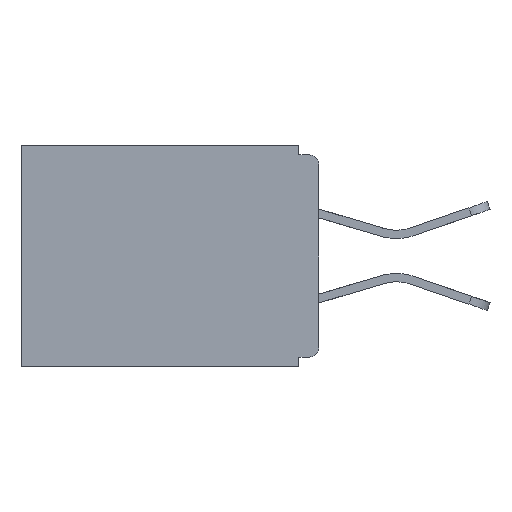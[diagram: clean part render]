
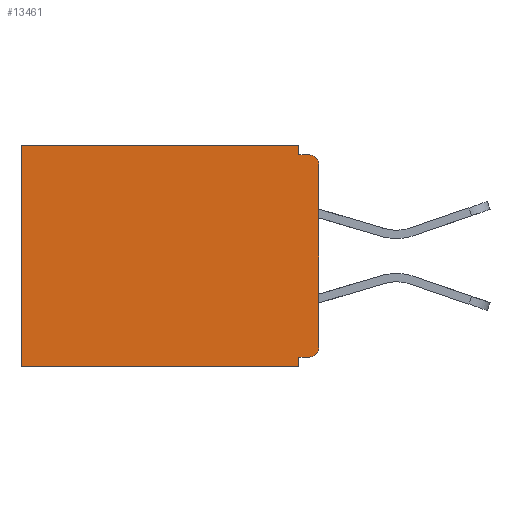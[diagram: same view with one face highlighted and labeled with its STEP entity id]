
A CAD part, left-side view. The second image highlights one B-rep face of the part: STEP entity #13461.
In plain terms, the highlighted planar face has unit normal (-1, 0, 0).
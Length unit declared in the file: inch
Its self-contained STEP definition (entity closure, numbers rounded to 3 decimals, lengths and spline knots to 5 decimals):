
#26 = CARTESIAN_POINT ( 'NONE',  ( 0.298, 0.031, -0.015 ) ) ;
#28 = CARTESIAN_POINT ( 'NONE',  ( 0.298, 0.031, -0.343 ) ) ;
#801 = ORIENTED_EDGE ( 'NONE', *, *, #3856, .F. ) ;
#1372 = CARTESIAN_POINT ( 'NONE',  ( 0.298, 0.015, -0.328 ) ) ;
#1725 = VERTEX_POINT ( 'NONE', #3124 ) ;
#2933 = LINE ( 'NONE', #20693, #17212 ) ;
#3124 = CARTESIAN_POINT ( 'NONE',  ( 0.298, 0., -0.313 ) ) ;
#3155 = DIRECTION ( 'NONE',  ( 1., 0., 0. ) ) ;
#3326 = DIRECTION ( 'NONE',  ( 0., 0., -1. ) ) ;
#3626 = ORIENTED_EDGE ( 'NONE', *, *, #18985, .F. ) ;
#3690 = LINE ( 'NONE', #6072, #11023 ) ;
#3773 = VERTEX_POINT ( 'NONE', #9510 ) ;
#3856 = EDGE_CURVE ( 'NONE', #18642, #16194, #2933, .T. ) ;
#3944 = CARTESIAN_POINT ( 'NONE',  ( 0.298, 0.46, 0. ) ) ;
#4284 = ORIENTED_EDGE ( 'NONE', *, *, #15803, .T. ) ;
#5026 = ORIENTED_EDGE ( 'NONE', *, *, #6242, .T. ) ;
#5992 = CARTESIAN_POINT ( 'NONE',  ( 0.298, 0.031, -0.328 ) ) ;
#6072 = CARTESIAN_POINT ( 'NONE',  ( 0.298, 0., -0.343 ) ) ;
#6242 = EDGE_CURVE ( 'NONE', #18642, #1725, #12892, .T. ) ;
#6780 = VECTOR ( 'NONE', #15890, 39.37008 ) ;
#7370 = LINE ( 'NONE', #23292, #15363 ) ;
#7506 = CARTESIAN_POINT ( 'NONE',  ( 0.298, 0.031, -0.343 ) ) ;
#8250 = AXIS2_PLACEMENT_3D ( 'NONE', #19083, #21010, #25500 ) ;
#8762 = ORIENTED_EDGE ( 'NONE', *, *, #12440, .T. ) ;
#9299 = CARTESIAN_POINT ( 'NONE',  ( 0.298, 0., 0. ) ) ;
#9510 = CARTESIAN_POINT ( 'NONE',  ( 0.298, 0.015, -0.015 ) ) ;
#9830 = EDGE_CURVE ( 'NONE', #27443, #1725, #27353, .T. ) ;
#9964 = VERTEX_POINT ( 'NONE', #25817 ) ;
#9993 = CARTESIAN_POINT ( 'NONE',  ( 0.298, 0.031, 0. ) ) ;
#10000 = CIRCLE ( 'NONE', #27553, 0.015 ) ;
#10158 = ORIENTED_EDGE ( 'NONE', *, *, #10792, .T. ) ;
#10476 = VECTOR ( 'NONE', #16691, 39.37008 ) ;
#10576 = AXIS2_PLACEMENT_3D ( 'NONE', #9299, #3155, #18013 ) ;
#10618 = DIRECTION ( 'NONE',  ( 0., 0., -1. ) ) ;
#10792 = EDGE_CURVE ( 'NONE', #27443, #3773, #10000, .T. ) ;
#10989 = VERTEX_POINT ( 'NONE', #3944 ) ;
#11023 = VECTOR ( 'NONE', #27179, 39.37008 ) ;
#11535 = PLANE ( 'NONE',  #10576 ) ;
#12085 = DIRECTION ( 'NONE',  ( -1., 0., 0. ) ) ;
#12440 = EDGE_CURVE ( 'NONE', #23164, #10989, #18532, .T. ) ;
#12633 = LINE ( 'NONE', #7506, #13975 ) ;
#12892 = CIRCLE ( 'NONE', #8250, 0.015 ) ;
#13461 = ADVANCED_FACE ( 'NONE', ( #26113 ), #11535, .F. ) ;
#13865 = CARTESIAN_POINT ( 'NONE',  ( 0.298, 0.015, -0.03 ) ) ;
#13975 = VECTOR ( 'NONE', #3326, 39.37008 ) ;
#14434 = LINE ( 'NONE', #26762, #6780 ) ;
#14671 = EDGE_CURVE ( 'NONE', #23164, #26048, #15767, .T. ) ;
#14679 = VERTEX_POINT ( 'NONE', #20923 ) ;
#15363 = VECTOR ( 'NONE', #10618, 39.37008 ) ;
#15387 = ORIENTED_EDGE ( 'NONE', *, *, #26949, .F. ) ;
#15547 = DIRECTION ( 'NONE',  ( 0., 1., 0. ) ) ;
#15767 = LINE ( 'NONE', #28, #10476 ) ;
#15803 = EDGE_CURVE ( 'NONE', #10989, #14679, #7370, .T. ) ;
#15890 = DIRECTION ( 'NONE',  ( 0., -1., 0. ) ) ;
#16194 = VERTEX_POINT ( 'NONE', #5992 ) ;
#16691 = DIRECTION ( 'NONE',  ( 0., 0., -1. ) ) ;
#17212 = VECTOR ( 'NONE', #18580, 39.37008 ) ;
#17706 = ORIENTED_EDGE ( 'NONE', *, *, #19653, .F. ) ;
#18013 = DIRECTION ( 'NONE',  ( 0., 0., -1. ) ) ;
#18305 = ORIENTED_EDGE ( 'NONE', *, *, #9830, .F. ) ;
#18532 = LINE ( 'NONE', #21848, #22827 ) ;
#18580 = DIRECTION ( 'NONE',  ( 0., 1., 0. ) ) ;
#18642 = VERTEX_POINT ( 'NONE', #1372 ) ;
#18931 = CARTESIAN_POINT ( 'NONE',  ( 0.298, 0., 0. ) ) ;
#18985 = EDGE_CURVE ( 'NONE', #9964, #14679, #3690, .T. ) ;
#19083 = CARTESIAN_POINT ( 'NONE',  ( 0.298, 0.015, -0.313 ) ) ;
#19653 = EDGE_CURVE ( 'NONE', #16194, #9964, #12633, .T. ) ;
#20693 = CARTESIAN_POINT ( 'NONE',  ( 0.298, 0., -0.328 ) ) ;
#20923 = CARTESIAN_POINT ( 'NONE',  ( 0.298, 0.46, -0.343 ) ) ;
#21010 = DIRECTION ( 'NONE',  ( -1., 0., 0. ) ) ;
#21139 = DIRECTION ( 'NONE',  ( 0., 0., -1. ) ) ;
#21320 = DIRECTION ( 'NONE',  ( 0., 0., -1. ) ) ;
#21848 = CARTESIAN_POINT ( 'NONE',  ( 0.298, 0., 0. ) ) ;
#22293 = ORIENTED_EDGE ( 'NONE', *, *, #14671, .F. ) ;
#22647 = VECTOR ( 'NONE', #21139, 39.37008 ) ;
#22827 = VECTOR ( 'NONE', #15547, 39.37008 ) ;
#23164 = VERTEX_POINT ( 'NONE', #9993 ) ;
#23292 = CARTESIAN_POINT ( 'NONE',  ( 0.298, 0.46, 0. ) ) ;
#23924 = CARTESIAN_POINT ( 'NONE',  ( 0.298, 0., -0.03 ) ) ;
#25500 = DIRECTION ( 'NONE',  ( 0., 0., -1. ) ) ;
#25817 = CARTESIAN_POINT ( 'NONE',  ( 0.298, 0.031, -0.343 ) ) ;
#26048 = VERTEX_POINT ( 'NONE', #26 ) ;
#26113 = FACE_OUTER_BOUND ( 'NONE', #27386, .T. ) ;
#26762 = CARTESIAN_POINT ( 'NONE',  ( 0.298, 0., -0.015 ) ) ;
#26949 = EDGE_CURVE ( 'NONE', #26048, #3773, #14434, .T. ) ;
#27179 = DIRECTION ( 'NONE',  ( 0., 1., 0. ) ) ;
#27353 = LINE ( 'NONE', #18931, #22647 ) ;
#27386 = EDGE_LOOP ( 'NONE', ( #10158, #15387, #22293, #8762, #4284, #3626, #17706, #801, #5026, #18305 ) ) ;
#27443 = VERTEX_POINT ( 'NONE', #23924 ) ;
#27553 = AXIS2_PLACEMENT_3D ( 'NONE', #13865, #12085, #21320 ) ;
